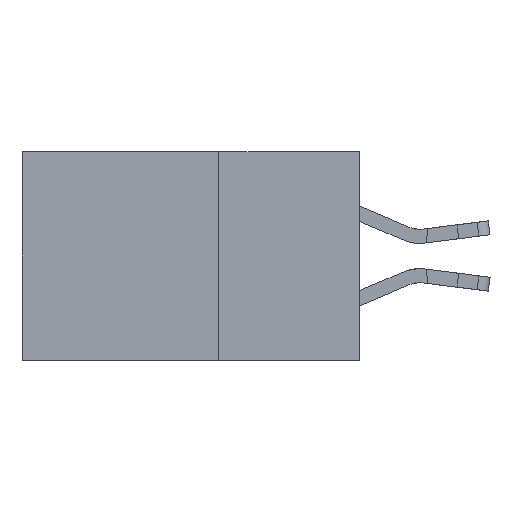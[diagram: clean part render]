
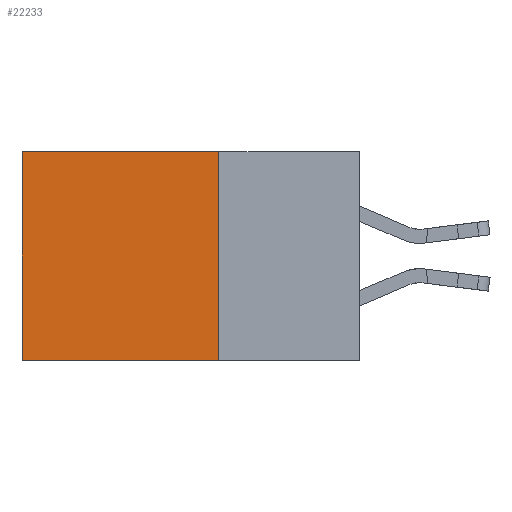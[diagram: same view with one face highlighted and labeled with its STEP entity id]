
A CAD part, left-side view. The second image highlights one B-rep face of the part: STEP entity #22233.
In plain terms, the highlighted planar face has unit normal (-1, 0, 0).
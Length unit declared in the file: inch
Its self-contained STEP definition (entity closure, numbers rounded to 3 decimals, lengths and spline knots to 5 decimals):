
#199 = CARTESIAN_POINT ( 'NONE',  ( 0.2875, 0.6, 0. ) ) ;
#442 = LINE ( 'NONE', #28980, #6179 ) ;
#468 = ORIENTED_EDGE ( 'NONE', *, *, #10311, .F. ) ;
#864 = DIRECTION ( 'NONE',  ( 1., 0., 0. ) ) ;
#1742 = ORIENTED_EDGE ( 'NONE', *, *, #18181, .T. ) ;
#3371 = CARTESIAN_POINT ( 'NONE',  ( 0.2875, 0.25, 0. ) ) ;
#3395 = LINE ( 'NONE', #199, #31078 ) ;
#3718 = PLANE ( 'NONE',  #16790 ) ;
#4112 = VERTEX_POINT ( 'NONE', #10000 ) ;
#4839 = VERTEX_POINT ( 'NONE', #10749 ) ;
#6179 = VECTOR ( 'NONE', #15618, 39.37008 ) ;
#6319 = DIRECTION ( 'NONE',  ( 0., 0., -1. ) ) ;
#7289 = EDGE_CURVE ( 'NONE', #18841, #30630, #3395, .T. ) ;
#10000 = CARTESIAN_POINT ( 'NONE',  ( 0.2875, 0.25, -0.37 ) ) ;
#10311 = EDGE_CURVE ( 'NONE', #4112, #30630, #11295, .T. ) ;
#10389 = DIRECTION ( 'NONE',  ( 0., 1., 0. ) ) ;
#10749 = CARTESIAN_POINT ( 'NONE',  ( 0.2875, 0.25, 0. ) ) ;
#11295 = LINE ( 'NONE', #23163, #13238 ) ;
#11807 = DIRECTION ( 'NONE',  ( 0., 0., -1. ) ) ;
#13139 = ORIENTED_EDGE ( 'NONE', *, *, #7289, .T. ) ;
#13238 = VECTOR ( 'NONE', #10389, 39.37008 ) ;
#14263 = FACE_OUTER_BOUND ( 'NONE', #22104, .T. ) ;
#15124 = EDGE_CURVE ( 'NONE', #4839, #4112, #27994, .T. ) ;
#15618 = DIRECTION ( 'NONE',  ( 0., 1., 0. ) ) ;
#16790 = AXIS2_PLACEMENT_3D ( 'NONE', #3371, #864, #6319 ) ;
#18181 = EDGE_CURVE ( 'NONE', #4839, #18841, #442, .T. ) ;
#18841 = VERTEX_POINT ( 'NONE', #21689 ) ;
#21689 = CARTESIAN_POINT ( 'NONE',  ( 0.2875, 0.6, 0. ) ) ;
#22104 = EDGE_LOOP ( 'NONE', ( #13139, #468, #28219, #1742 ) ) ;
#22233 = ADVANCED_FACE ( 'NONE', ( #14263 ), #3718, .F. ) ;
#23163 = CARTESIAN_POINT ( 'NONE',  ( 0.2875, 0.25, -0.37 ) ) ;
#24347 = CARTESIAN_POINT ( 'NONE',  ( 0.2875, 0.6, -0.37 ) ) ;
#27994 = LINE ( 'NONE', #32452, #33171 ) ;
#28219 = ORIENTED_EDGE ( 'NONE', *, *, #15124, .F. ) ;
#28980 = CARTESIAN_POINT ( 'NONE',  ( 0.2875, 0.25, 0. ) ) ;
#30630 = VERTEX_POINT ( 'NONE', #24347 ) ;
#31078 = VECTOR ( 'NONE', #33263, 39.37008 ) ;
#32452 = CARTESIAN_POINT ( 'NONE',  ( 0.2875, 0.25, 0. ) ) ;
#33171 = VECTOR ( 'NONE', #11807, 39.37008 ) ;
#33263 = DIRECTION ( 'NONE',  ( 0., 0., -1. ) ) ;
